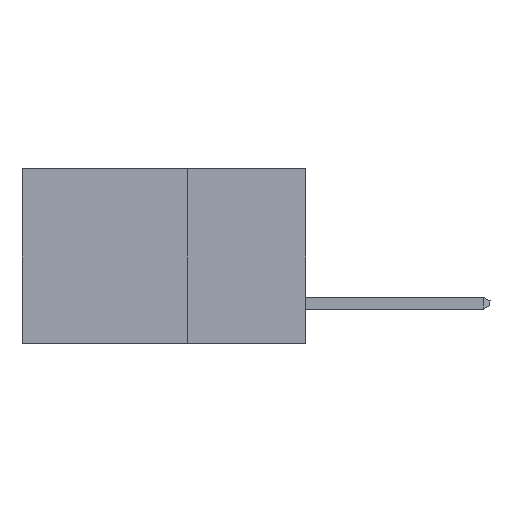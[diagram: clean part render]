
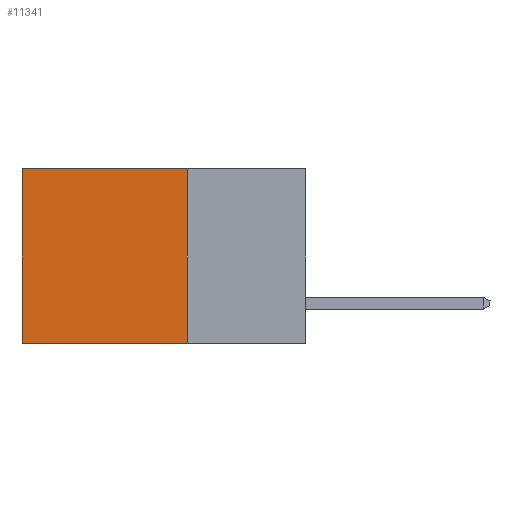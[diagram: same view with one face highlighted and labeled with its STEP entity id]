
A CAD part, left-side view. The second image highlights one B-rep face of the part: STEP entity #11341.
In plain terms, the highlighted planar face has unit normal (-1, 0, 0).
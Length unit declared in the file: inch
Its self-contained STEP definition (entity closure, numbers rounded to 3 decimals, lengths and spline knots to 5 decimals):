
#120 = EDGE_CURVE ( 'NONE', #2797, #9529, #6761, .T. ) ;
#550 = EDGE_CURVE ( 'NONE', #11222, #2797, #906, .T. ) ;
#618 = CARTESIAN_POINT ( 'NONE',  ( 0.2615, 0.6, 0. ) ) ;
#906 = LINE ( 'NONE', #8829, #12140 ) ;
#1333 = ORIENTED_EDGE ( 'NONE', *, *, #120, .F. ) ;
#2036 = CARTESIAN_POINT ( 'NONE',  ( 0.2615, 0.25, 0. ) ) ;
#2564 = LINE ( 'NONE', #5575, #4425 ) ;
#2797 = VERTEX_POINT ( 'NONE', #4200 ) ;
#2919 = EDGE_CURVE ( 'NONE', #11222, #6545, #2564, .T. ) ;
#3293 = CARTESIAN_POINT ( 'NONE',  ( 0.2615, 0.6, -0.37 ) ) ;
#4121 = AXIS2_PLACEMENT_3D ( 'NONE', #6483, #10475, #12502 ) ;
#4200 = CARTESIAN_POINT ( 'NONE',  ( 0.2615, 0.25, -0.37 ) ) ;
#4415 = ORIENTED_EDGE ( 'NONE', *, *, #6535, .T. ) ;
#4425 = VECTOR ( 'NONE', #8334, 39.37008 ) ;
#4499 = ORIENTED_EDGE ( 'NONE', *, *, #2919, .T. ) ;
#5306 = FACE_OUTER_BOUND ( 'NONE', #8927, .T. ) ;
#5575 = CARTESIAN_POINT ( 'NONE',  ( 0.2615, 0.25, 0. ) ) ;
#5586 = CARTESIAN_POINT ( 'NONE',  ( 0.2615, 0.6, -0.37 ) ) ;
#6483 = CARTESIAN_POINT ( 'NONE',  ( 0.2615, 0.25, -0.37 ) ) ;
#6535 = EDGE_CURVE ( 'NONE', #6545, #9529, #6637, .T. ) ;
#6545 = VERTEX_POINT ( 'NONE', #618 ) ;
#6637 = LINE ( 'NONE', #5586, #6991 ) ;
#6761 = LINE ( 'NONE', #8924, #6896 ) ;
#6896 = VECTOR ( 'NONE', #8073, 39.37008 ) ;
#6991 = VECTOR ( 'NONE', #9588, 39.37008 ) ;
#7405 = PLANE ( 'NONE',  #4121 ) ;
#8073 = DIRECTION ( 'NONE',  ( 0., 1., 0. ) ) ;
#8334 = DIRECTION ( 'NONE',  ( 0., 1., 0. ) ) ;
#8829 = CARTESIAN_POINT ( 'NONE',  ( 0.2615, 0.25, -0.37 ) ) ;
#8924 = CARTESIAN_POINT ( 'NONE',  ( 0.2615, 0.25, -0.37 ) ) ;
#8927 = EDGE_LOOP ( 'NONE', ( #4415, #1333, #11472, #4499 ) ) ;
#9529 = VERTEX_POINT ( 'NONE', #3293 ) ;
#9588 = DIRECTION ( 'NONE',  ( 0., 0., -1. ) ) ;
#10475 = DIRECTION ( 'NONE',  ( 1., 0., 0. ) ) ;
#11222 = VERTEX_POINT ( 'NONE', #2036 ) ;
#11341 = ADVANCED_FACE ( 'NONE', ( #5306 ), #7405, .F. ) ;
#11472 = ORIENTED_EDGE ( 'NONE', *, *, #550, .F. ) ;
#12140 = VECTOR ( 'NONE', #12807, 39.37008 ) ;
#12502 = DIRECTION ( 'NONE',  ( 0., 0., -1. ) ) ;
#12807 = DIRECTION ( 'NONE',  ( 0., 0., -1. ) ) ;
